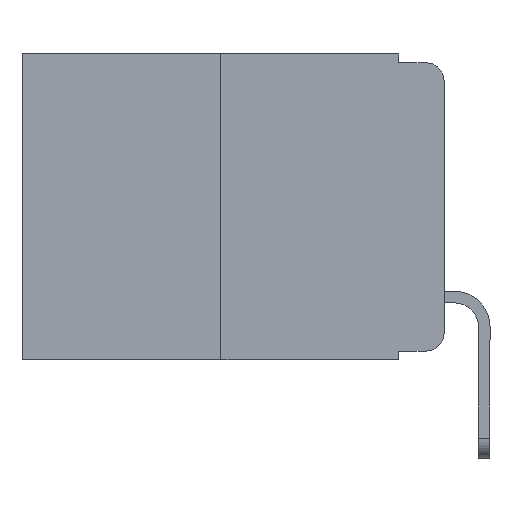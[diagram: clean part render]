
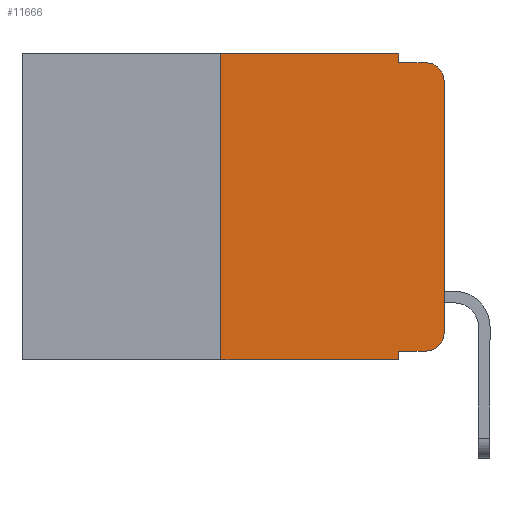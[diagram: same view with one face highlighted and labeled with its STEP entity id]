
A CAD part, left-side view. The second image highlights one B-rep face of the part: STEP entity #11666.
In plain terms, the highlighted planar face has unit normal (-1, 0, 0).
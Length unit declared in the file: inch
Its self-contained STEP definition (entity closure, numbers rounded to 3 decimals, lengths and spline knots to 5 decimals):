
#321 = AXIS2_PLACEMENT_3D ( 'NONE', #876, #820, #3405 ) ;
#583 = LINE ( 'NONE', #9785, #3738 ) ;
#594 = VERTEX_POINT ( 'NONE', #11872 ) ;
#620 = LINE ( 'NONE', #7055, #10801 ) ;
#750 = ORIENTED_EDGE ( 'NONE', *, *, #2327, .T. ) ;
#758 = CARTESIAN_POINT ( 'NONE',  ( 0., 0., -0.313 ) ) ;
#779 = CARTESIAN_POINT ( 'NONE',  ( 0., 0.051, -0.01 ) ) ;
#812 = DIRECTION ( 'NONE',  ( 0., 0., -1. ) ) ;
#820 = DIRECTION ( 'NONE',  ( -1., 0., 0. ) ) ;
#876 = CARTESIAN_POINT ( 'NONE',  ( 0., 0.02, -0.03 ) ) ;
#898 = EDGE_CURVE ( 'NONE', #9850, #1891, #583, .T. ) ;
#947 = EDGE_LOOP ( 'NONE', ( #1110, #1455, #2131, #12502, #1309, #7032, #7664, #5572, #5891, #750 ) ) ;
#996 = CARTESIAN_POINT ( 'NONE',  ( 0., 0.051, -0.343 ) ) ;
#1110 = ORIENTED_EDGE ( 'NONE', *, *, #4752, .T. ) ;
#1309 = ORIENTED_EDGE ( 'NONE', *, *, #6685, .F. ) ;
#1331 = CARTESIAN_POINT ( 'NONE',  ( 0., 0.25, -0.343 ) ) ;
#1421 = AXIS2_PLACEMENT_3D ( 'NONE', #6299, #2311, #9206 ) ;
#1455 = ORIENTED_EDGE ( 'NONE', *, *, #3501, .T. ) ;
#1519 = AXIS2_PLACEMENT_3D ( 'NONE', #5509, #5488, #5468 ) ;
#1873 = CARTESIAN_POINT ( 'NONE',  ( 0., 0.051, -0.333 ) ) ;
#1891 = VERTEX_POINT ( 'NONE', #996 ) ;
#2004 = VECTOR ( 'NONE', #4011, 39.37008 ) ;
#2094 = DIRECTION ( 'NONE',  ( 0., -1., 0. ) ) ;
#2131 = ORIENTED_EDGE ( 'NONE', *, *, #8333, .F. ) ;
#2311 = DIRECTION ( 'NONE',  ( 1., 0., 0. ) ) ;
#2327 = EDGE_CURVE ( 'NONE', #4915, #11474, #6356, .T. ) ;
#2524 = CARTESIAN_POINT ( 'NONE',  ( 0., 0.473, 0. ) ) ;
#2548 = VERTEX_POINT ( 'NONE', #4183 ) ;
#2578 = CIRCLE ( 'NONE', #321, 0.02 ) ;
#2703 = LINE ( 'NONE', #779, #10114 ) ;
#3017 = EDGE_CURVE ( 'NONE', #594, #4915, #12582, .T. ) ;
#3083 = CARTESIAN_POINT ( 'NONE',  ( 0., 0.02, -0.333 ) ) ;
#3120 = VECTOR ( 'NONE', #6919, 39.37008 ) ;
#3405 = DIRECTION ( 'NONE',  ( 0., 0., -1. ) ) ;
#3501 = EDGE_CURVE ( 'NONE', #2548, #6309, #2578, .T. ) ;
#3738 = VECTOR ( 'NONE', #9811, 39.37008 ) ;
#3853 = CARTESIAN_POINT ( 'NONE',  ( 0., 0.25, 0. ) ) ;
#4011 = DIRECTION ( 'NONE',  ( 0., 0., -1. ) ) ;
#4183 = CARTESIAN_POINT ( 'NONE',  ( 0., 0., -0.03 ) ) ;
#4199 = DIRECTION ( 'NONE',  ( 0., 0., 1. ) ) ;
#4216 = VERTEX_POINT ( 'NONE', #11507 ) ;
#4752 = EDGE_CURVE ( 'NONE', #11474, #2548, #620, .T. ) ;
#4915 = VERTEX_POINT ( 'NONE', #3083 ) ;
#5411 = LINE ( 'NONE', #2524, #10757 ) ;
#5468 = DIRECTION ( 'NONE',  ( 0., 0., -1. ) ) ;
#5488 = DIRECTION ( 'NONE',  ( -1., 0., 0. ) ) ;
#5509 = CARTESIAN_POINT ( 'NONE',  ( 0., 0.02, -0.313 ) ) ;
#5572 = ORIENTED_EDGE ( 'NONE', *, *, #7041, .F. ) ;
#5717 = LINE ( 'NONE', #3853, #3120 ) ;
#5891 = ORIENTED_EDGE ( 'NONE', *, *, #3017, .T. ) ;
#6299 = CARTESIAN_POINT ( 'NONE',  ( 0., 0.473, 0. ) ) ;
#6309 = VERTEX_POINT ( 'NONE', #9856 ) ;
#6356 = CIRCLE ( 'NONE', #1519, 0.02 ) ;
#6685 = EDGE_CURVE ( 'NONE', #4216, #7151, #5411, .T. ) ;
#6919 = DIRECTION ( 'NONE',  ( 0., 0., 1. ) ) ;
#7032 = ORIENTED_EDGE ( 'NONE', *, *, #7714, .F. ) ;
#7041 = EDGE_CURVE ( 'NONE', #594, #1891, #7669, .T. ) ;
#7055 = CARTESIAN_POINT ( 'NONE',  ( 0., 0., 0. ) ) ;
#7151 = VERTEX_POINT ( 'NONE', #10733 ) ;
#7322 = PLANE ( 'NONE',  #1421 ) ;
#7664 = ORIENTED_EDGE ( 'NONE', *, *, #898, .T. ) ;
#7669 = LINE ( 'NONE', #12354, #12113 ) ;
#7714 = EDGE_CURVE ( 'NONE', #9850, #4216, #5717, .T. ) ;
#8333 = EDGE_CURVE ( 'NONE', #10914, #6309, #2703, .T. ) ;
#8373 = EDGE_CURVE ( 'NONE', #7151, #10914, #12409, .T. ) ;
#8946 = FACE_OUTER_BOUND ( 'NONE', #947, .T. ) ;
#8954 = CARTESIAN_POINT ( 'NONE',  ( 0., 0.051, 0. ) ) ;
#9206 = DIRECTION ( 'NONE',  ( 0., 0., -1. ) ) ;
#9371 = DIRECTION ( 'NONE',  ( 0., -1., 0. ) ) ;
#9785 = CARTESIAN_POINT ( 'NONE',  ( 0., 0.473, -0.343 ) ) ;
#9811 = DIRECTION ( 'NONE',  ( 0., -1., 0. ) ) ;
#9850 = VERTEX_POINT ( 'NONE', #1331 ) ;
#9856 = CARTESIAN_POINT ( 'NONE',  ( 0., 0.02, -0.01 ) ) ;
#10114 = VECTOR ( 'NONE', #12368, 39.37008 ) ;
#10733 = CARTESIAN_POINT ( 'NONE',  ( 0., 0.051, 0. ) ) ;
#10757 = VECTOR ( 'NONE', #9371, 39.37008 ) ;
#10801 = VECTOR ( 'NONE', #4199, 39.37008 ) ;
#10914 = VERTEX_POINT ( 'NONE', #11579 ) ;
#11474 = VERTEX_POINT ( 'NONE', #758 ) ;
#11507 = CARTESIAN_POINT ( 'NONE',  ( 0., 0.25, 0. ) ) ;
#11579 = CARTESIAN_POINT ( 'NONE',  ( 0., 0.051, -0.01 ) ) ;
#11666 = ADVANCED_FACE ( 'NONE', ( #8946 ), #7322, .F. ) ;
#11872 = CARTESIAN_POINT ( 'NONE',  ( 0., 0.051, -0.333 ) ) ;
#12113 = VECTOR ( 'NONE', #812, 39.37008 ) ;
#12312 = VECTOR ( 'NONE', #2094, 39.37008 ) ;
#12354 = CARTESIAN_POINT ( 'NONE',  ( 0., 0.051, 0. ) ) ;
#12368 = DIRECTION ( 'NONE',  ( 0., -1., 0. ) ) ;
#12409 = LINE ( 'NONE', #8954, #2004 ) ;
#12502 = ORIENTED_EDGE ( 'NONE', *, *, #8373, .F. ) ;
#12582 = LINE ( 'NONE', #1873, #12312 ) ;
